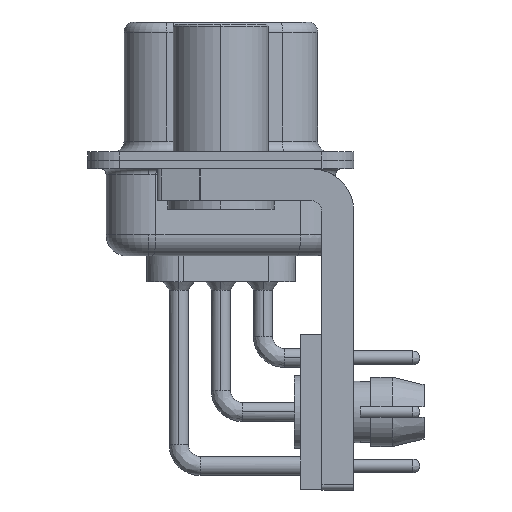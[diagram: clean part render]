
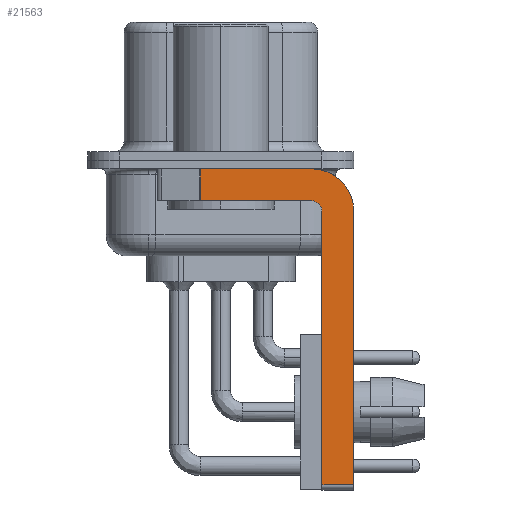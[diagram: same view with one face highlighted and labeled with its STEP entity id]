
A CAD part, left-side view. The second image highlights one B-rep face of the part: STEP entity #21563.
In plain terms, the highlighted planar face has unit normal (-1, 0, 0).
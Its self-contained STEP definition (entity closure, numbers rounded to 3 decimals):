
#599 = DIRECTION ( 'NONE',  ( 0., -1., 0. ) ) ;
#1063 = LINE ( 'NONE', #1432, #21448 ) ;
#1432 = CARTESIAN_POINT ( 'NONE',  ( -2.9, -6.25, -2.4 ) ) ;
#1721 = ORIENTED_EDGE ( 'NONE', *, *, #32190, .T. ) ;
#2084 = CARTESIAN_POINT ( 'NONE',  ( -2.9, 0.978, -0.4 ) ) ;
#2332 = ORIENTED_EDGE ( 'NONE', *, *, #33803, .F. ) ;
#3066 = EDGE_CURVE ( 'NONE', #16514, #14791, #20263, .T. ) ;
#3648 = DIRECTION ( 'NONE',  ( -1., 0., 0. ) ) ;
#3699 = LINE ( 'NONE', #33760, #24471 ) ;
#3916 = ORIENTED_EDGE ( 'NONE', *, *, #28265, .F. ) ;
#4434 = ORIENTED_EDGE ( 'NONE', *, *, #3066, .F. ) ;
#4454 = LINE ( 'NONE', #24376, #18587 ) ;
#4696 = PLANE ( 'NONE',  #5456 ) ;
#5456 = AXIS2_PLACEMENT_3D ( 'NONE', #15223, #7350, #25899 ) ;
#6214 = CARTESIAN_POINT ( 'NONE',  ( -2.9, -4.25, -2.4 ) ) ;
#7350 = DIRECTION ( 'NONE',  ( 1., 0., 0. ) ) ;
#8452 = ORIENTED_EDGE ( 'NONE', *, *, #30756, .F. ) ;
#8610 = LINE ( 'NONE', #32295, #21894 ) ;
#8704 = VERTEX_POINT ( 'NONE', #11901 ) ;
#8847 = DIRECTION ( 'NONE',  ( 0., 0., -1. ) ) ;
#8866 = ORIENTED_EDGE ( 'NONE', *, *, #17550, .F. ) ;
#8926 = CIRCLE ( 'NONE', #12579, 2. ) ;
#9004 = CARTESIAN_POINT ( 'NONE',  ( -2.9, -4.25, -1.9 ) ) ;
#9278 = ORIENTED_EDGE ( 'NONE', *, *, #15129, .T. ) ;
#11109 = DIRECTION ( 'NONE',  ( 0., 0., 1. ) ) ;
#11568 = AXIS2_PLACEMENT_3D ( 'NONE', #19545, #3648, #22195 ) ;
#11901 = CARTESIAN_POINT ( 'NONE',  ( -2.9, -4.25, -1.9 ) ) ;
#12555 = DIRECTION ( 'NONE',  ( 0., 0., -1. ) ) ;
#12579 = AXIS2_PLACEMENT_3D ( 'NONE', #6214, #24713, #8847 ) ;
#13144 = CIRCLE ( 'NONE', #11568, 0.5 ) ;
#14791 = VERTEX_POINT ( 'NONE', #21880 ) ;
#14978 = VECTOR ( 'NONE', #19701, 1000. ) ;
#15129 = EDGE_CURVE ( 'NONE', #16514, #20094, #3699, .T. ) ;
#15223 = CARTESIAN_POINT ( 'NONE',  ( -2.9, -4.25, -2.4 ) ) ;
#15547 = CARTESIAN_POINT ( 'NONE',  ( -2.9, -4.75, -2.4 ) ) ;
#16514 = VERTEX_POINT ( 'NONE', #2084 ) ;
#17094 = CARTESIAN_POINT ( 'NONE',  ( -2.9, 0.978, -1.9 ) ) ;
#17550 = EDGE_CURVE ( 'NONE', #31281, #31399, #1063, .T. ) ;
#17622 = CARTESIAN_POINT ( 'NONE',  ( -2.9, -6.25, -2.4 ) ) ;
#18587 = VECTOR ( 'NONE', #599, 1000. ) ;
#19545 = CARTESIAN_POINT ( 'NONE',  ( -2.9, -4.25, -2.4 ) ) ;
#19569 = LINE ( 'NONE', #9004, #14978 ) ;
#19701 = DIRECTION ( 'NONE',  ( 0., 1., 0. ) ) ;
#20021 = DIRECTION ( 'NONE',  ( 0., 0., -1. ) ) ;
#20094 = VERTEX_POINT ( 'NONE', #17094 ) ;
#20263 = LINE ( 'NONE', #22145, #33514 ) ;
#21408 = EDGE_LOOP ( 'NONE', ( #4434, #9278, #3916, #2332, #8452, #1721, #8866, #28615 ) ) ;
#21448 = VECTOR ( 'NONE', #20021, 1000. ) ;
#21563 = ADVANCED_FACE ( 'NONE', ( #28540 ), #4696, .F. ) ;
#21880 = CARTESIAN_POINT ( 'NONE',  ( -2.9, -4.25, -0.4 ) ) ;
#21894 = VECTOR ( 'NONE', #11109, 1000. ) ;
#22145 = CARTESIAN_POINT ( 'NONE',  ( -2.9, 3., -0.4 ) ) ;
#22195 = DIRECTION ( 'NONE',  ( 0., 0., 1. ) ) ;
#23631 = EDGE_CURVE ( 'NONE', #14791, #31281, #8926, .T. ) ;
#24376 = CARTESIAN_POINT ( 'NONE',  ( -2.9, -4.25, -15.25 ) ) ;
#24471 = VECTOR ( 'NONE', #12555, 1000. ) ;
#24713 = DIRECTION ( 'NONE',  ( 1., 0., 0. ) ) ;
#25899 = DIRECTION ( 'NONE',  ( 0., 0., -1. ) ) ;
#26887 = CARTESIAN_POINT ( 'NONE',  ( -2.9, -4.75, -15.25 ) ) ;
#28091 = VERTEX_POINT ( 'NONE', #26887 ) ;
#28265 = EDGE_CURVE ( 'NONE', #8704, #20094, #19569, .T. ) ;
#28540 = FACE_OUTER_BOUND ( 'NONE', #21408, .T. ) ;
#28615 = ORIENTED_EDGE ( 'NONE', *, *, #23631, .F. ) ;
#30756 = EDGE_CURVE ( 'NONE', #28091, #32588, #8610, .T. ) ;
#31259 = CARTESIAN_POINT ( 'NONE',  ( -2.9, -6.25, -15.25 ) ) ;
#31281 = VERTEX_POINT ( 'NONE', #17622 ) ;
#31399 = VERTEX_POINT ( 'NONE', #31259 ) ;
#32130 = DIRECTION ( 'NONE',  ( 0., -1., 0. ) ) ;
#32190 = EDGE_CURVE ( 'NONE', #28091, #31399, #4454, .T. ) ;
#32295 = CARTESIAN_POINT ( 'NONE',  ( -2.9, -4.75, -15.5 ) ) ;
#32588 = VERTEX_POINT ( 'NONE', #15547 ) ;
#33514 = VECTOR ( 'NONE', #32130, 1000. ) ;
#33760 = CARTESIAN_POINT ( 'NONE',  ( -2.9, 0.978, -1.9 ) ) ;
#33803 = EDGE_CURVE ( 'NONE', #32588, #8704, #13144, .T. ) ;
